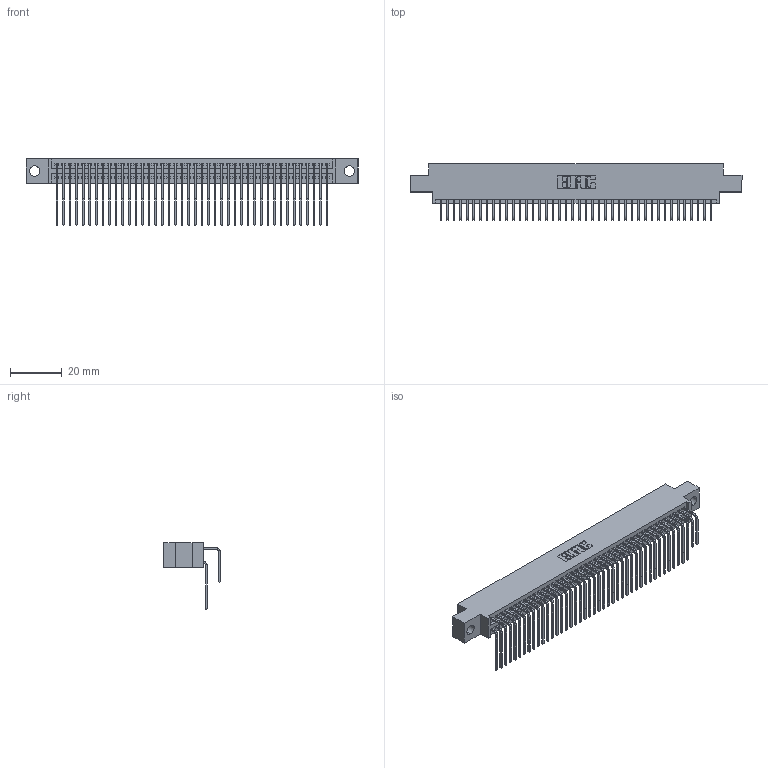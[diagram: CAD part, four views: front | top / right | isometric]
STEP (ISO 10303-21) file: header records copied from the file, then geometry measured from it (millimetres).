
FILE_DESCRIPTION (( 'STEP AP203' ), '1' );
FILE_NAME ('345-084-558-804.STEP', '2021-05-20T13:01:06', ( '' ), ( '' ), 'SwSTEP 2.0', 'SolidWorks 2020', '' );
FILE_SCHEMA (( 'CONFIG_CONTROL_DESIGN' ));
Length unit declared in the file: inch
Products named in the file (4): 345-292-001_558 559 Tail - 1; 345-084-558-804; 345 Part_0.170 Offset - 0.156 Dia-TI; 345-292-001_558 Tail - 2
Assembly tree (85 placements, depth 2):
  345-084-558-804
    345 Part_0.170 Offset - 0.156 Dia-TI
    345-292-001_558 559 Tail - 1  x42
    345-292-001_558 Tail - 2  x42
Bounding box: 127.89 x 21.83 x 25.53 mm (x, y, z)
Volume: 12688.5 mm3; surface area: 21029.4 mm2
Topology: 85 solids, 85 shells, 4512 faces, 13409 edges, 8826 vertices
Faces by surface type: plane 3038, cylinder 1474
Entity records: 35157 total; most frequent: CARTESIAN_POINT 5945, ORIENTED_EDGE 5826, DIRECTION 5213, EDGE_CURVE 2913, LINE 2573, VECTOR 2573, VERTEX_POINT 1938, AXIS2_PLACEMENT_3D 1320
